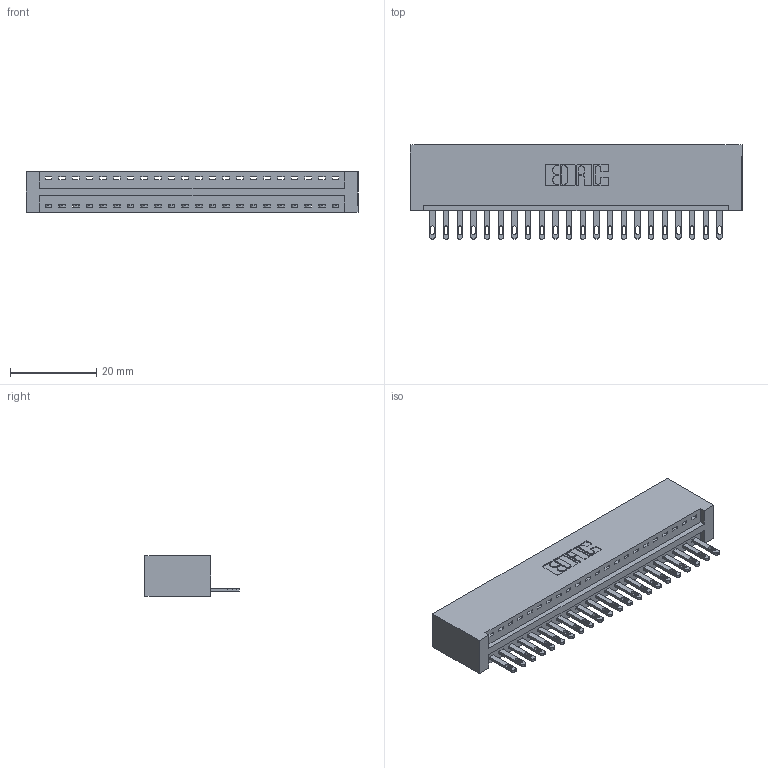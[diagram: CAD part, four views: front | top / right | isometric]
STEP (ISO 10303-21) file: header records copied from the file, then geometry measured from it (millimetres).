
FILE_DESCRIPTION (( 'STEP AP203' ), '1' );
FILE_NAME ('346-022-500-101.STEP', '2018-08-20T23:26:14', ( '' ), ( '' ), 'SwSTEP 2.0', 'SolidWorks 2016', '' );
FILE_SCHEMA (( 'CONFIG_CONTROL_DESIGN' ));
Length unit declared in the file: inch
Products named in the file (3): 346 Part_No Mounting Lugs; 345-292-001_345-293-100; 346-022-500-101
Assembly tree (23 placements, depth 2):
  346-022-500-101
    346 Part_No Mounting Lugs
    345-292-001_345-293-100  x22
Bounding box: 77.09 x 21.84 x 9.4 mm (x, y, z)
Volume: 7804.4 mm3; surface area: 9665 mm2
Topology: 23 solids, 23 shells, 1302 faces, 4001 edges, 2666 vertices
Faces by surface type: plane 820, cylinder 482
Entity records: 15999 total; most frequent: CARTESIAN_POINT 2754, ORIENTED_EDGE 2710, DIRECTION 2451, EDGE_CURVE 1355, VECTOR 1139, LINE 1139, VERTEX_POINT 902, AXIS2_PLACEMENT_3D 656
